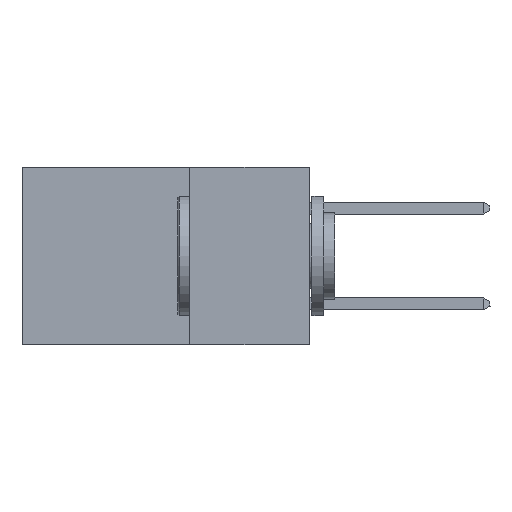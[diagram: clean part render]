
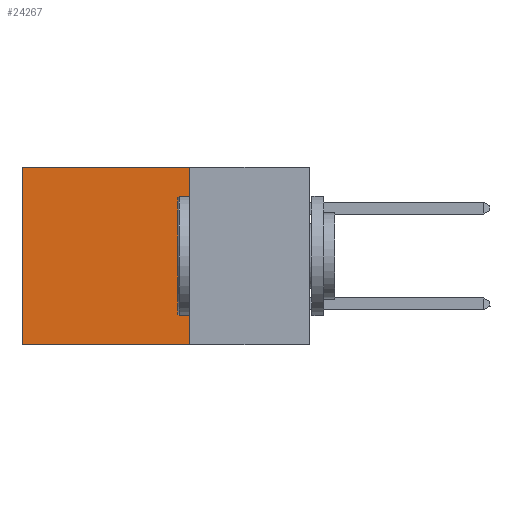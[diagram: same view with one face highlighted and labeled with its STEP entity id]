
A CAD part, left-side view. The second image highlights one B-rep face of the part: STEP entity #24267.
In plain terms, the highlighted planar face has unit normal (-1, 0, 0).
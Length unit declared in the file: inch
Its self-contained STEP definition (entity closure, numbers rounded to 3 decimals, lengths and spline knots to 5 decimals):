
#190 = CARTESIAN_POINT ( 'NONE',  ( 0.2875, 0.25, -0.37 ) ) ;
#1158 = EDGE_LOOP ( 'NONE', ( #29418, #5841, #8674, #29573 ) ) ;
#3453 = DIRECTION ( 'NONE',  ( 0., 0., -1. ) ) ;
#4012 = LINE ( 'NONE', #17665, #4399 ) ;
#4399 = VECTOR ( 'NONE', #15407, 39.37008 ) ;
#5510 = CARTESIAN_POINT ( 'NONE',  ( 0.2875, 0.25, 0. ) ) ;
#5841 = ORIENTED_EDGE ( 'NONE', *, *, #22025, .F. ) ;
#7658 = VERTEX_POINT ( 'NONE', #190 ) ;
#8674 = ORIENTED_EDGE ( 'NONE', *, *, #24319, .F. ) ;
#9357 = PLANE ( 'NONE',  #27598 ) ;
#11207 = VERTEX_POINT ( 'NONE', #5510 ) ;
#11665 = LINE ( 'NONE', #28177, #20848 ) ;
#11832 = CARTESIAN_POINT ( 'NONE',  ( 0.2875, 0.25, 0. ) ) ;
#11891 = CARTESIAN_POINT ( 'NONE',  ( 0.2875, 0.6, 0. ) ) ;
#12949 = DIRECTION ( 'NONE',  ( 0., 1., 0. ) ) ;
#14451 = CARTESIAN_POINT ( 'NONE',  ( 0.2875, 0.6, 0. ) ) ;
#15407 = DIRECTION ( 'NONE',  ( 0., 1., 0. ) ) ;
#15938 = VERTEX_POINT ( 'NONE', #29309 ) ;
#16750 = DIRECTION ( 'NONE',  ( 0., 0., -1. ) ) ;
#17665 = CARTESIAN_POINT ( 'NONE',  ( 0.2875, 0.25, 0. ) ) ;
#17890 = FACE_OUTER_BOUND ( 'NONE', #1158, .T. ) ;
#19848 = VECTOR ( 'NONE', #23170, 39.37008 ) ;
#20736 = VERTEX_POINT ( 'NONE', #11891 ) ;
#20848 = VECTOR ( 'NONE', #12949, 39.37008 ) ;
#21878 = VECTOR ( 'NONE', #16750, 39.37008 ) ;
#22025 = EDGE_CURVE ( 'NONE', #7658, #15938, #11665, .T. ) ;
#23170 = DIRECTION ( 'NONE',  ( 0., 0., -1. ) ) ;
#23250 = EDGE_CURVE ( 'NONE', #11207, #20736, #4012, .T. ) ;
#24267 = ADVANCED_FACE ( 'NONE', ( #17890 ), #9357, .F. ) ;
#24319 = EDGE_CURVE ( 'NONE', #11207, #7658, #30999, .T. ) ;
#25013 = EDGE_CURVE ( 'NONE', #20736, #15938, #26541, .T. ) ;
#26541 = LINE ( 'NONE', #14451, #19848 ) ;
#27598 = AXIS2_PLACEMENT_3D ( 'NONE', #11832, #29638, #3453 ) ;
#28177 = CARTESIAN_POINT ( 'NONE',  ( 0.2875, 0.25, -0.37 ) ) ;
#29309 = CARTESIAN_POINT ( 'NONE',  ( 0.2875, 0.6, -0.37 ) ) ;
#29418 = ORIENTED_EDGE ( 'NONE', *, *, #25013, .T. ) ;
#29573 = ORIENTED_EDGE ( 'NONE', *, *, #23250, .T. ) ;
#29638 = DIRECTION ( 'NONE',  ( 1., 0., 0. ) ) ;
#30999 = LINE ( 'NONE', #31400, #21878 ) ;
#31400 = CARTESIAN_POINT ( 'NONE',  ( 0.2875, 0.25, 0. ) ) ;
